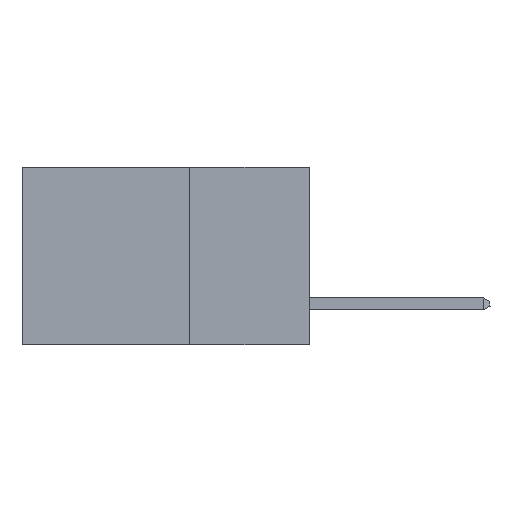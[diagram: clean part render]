
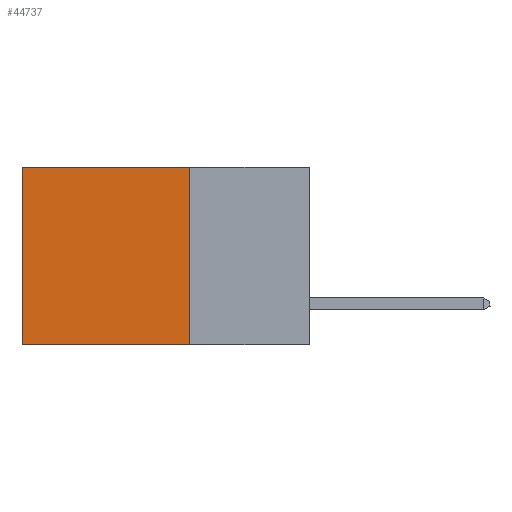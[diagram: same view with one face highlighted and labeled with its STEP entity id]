
A CAD part, left-side view. The second image highlights one B-rep face of the part: STEP entity #44737.
In plain terms, the highlighted planar face has unit normal (-1, 0, 0).
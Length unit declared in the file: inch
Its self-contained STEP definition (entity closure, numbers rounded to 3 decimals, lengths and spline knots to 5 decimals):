
#34 = VERTEX_POINT ( 'NONE', #30657 ) ;
#1559 = CARTESIAN_POINT ( 'NONE',  ( 0.2875, 0.25, 0. ) ) ;
#3124 = CARTESIAN_POINT ( 'NONE',  ( 0.2875, 0.6, -0.37 ) ) ;
#3145 = CARTESIAN_POINT ( 'NONE',  ( 0.2875, 0.6, 0. ) ) ;
#5218 = LINE ( 'NONE', #1559, #32919 ) ;
#6245 = VERTEX_POINT ( 'NONE', #25304 ) ;
#6445 = DIRECTION ( 'NONE',  ( 0., 0., -1. ) ) ;
#10493 = PLANE ( 'NONE',  #23070 ) ;
#14621 = DIRECTION ( 'NONE',  ( 1., 0., 0. ) ) ;
#14644 = DIRECTION ( 'NONE',  ( 0., 1., 0. ) ) ;
#15422 = VECTOR ( 'NONE', #6445, 39.37008 ) ;
#15622 = VECTOR ( 'NONE', #14644, 39.37008 ) ;
#15730 = ORIENTED_EDGE ( 'NONE', *, *, #23842, .F. ) ;
#17324 = CARTESIAN_POINT ( 'NONE',  ( 0.2875, 0.25, 0. ) ) ;
#18258 = CARTESIAN_POINT ( 'NONE',  ( 0.2875, 0.25, -0.37 ) ) ;
#18397 = DIRECTION ( 'NONE',  ( 0., 0., -1. ) ) ;
#21689 = ORIENTED_EDGE ( 'NONE', *, *, #38879, .F. ) ;
#21872 = LINE ( 'NONE', #29032, #15422 ) ;
#23070 = AXIS2_PLACEMENT_3D ( 'NONE', #37165, #14621, #18397 ) ;
#23842 = EDGE_CURVE ( 'NONE', #6245, #43455, #36805, .T. ) ;
#23954 = FACE_OUTER_BOUND ( 'NONE', #36875, .T. ) ;
#25304 = CARTESIAN_POINT ( 'NONE',  ( 0.2875, 0.25, -0.37 ) ) ;
#26646 = EDGE_CURVE ( 'NONE', #45426, #43455, #21872, .T. ) ;
#27005 = ORIENTED_EDGE ( 'NONE', *, *, #32850, .T. ) ;
#28950 = VECTOR ( 'NONE', #43688, 39.37008 ) ;
#29032 = CARTESIAN_POINT ( 'NONE',  ( 0.2875, 0.6, 0. ) ) ;
#30657 = CARTESIAN_POINT ( 'NONE',  ( 0.2875, 0.25, 0. ) ) ;
#32850 = EDGE_CURVE ( 'NONE', #34, #45426, #5218, .T. ) ;
#32919 = VECTOR ( 'NONE', #38872, 39.37008 ) ;
#36805 = LINE ( 'NONE', #18258, #15622 ) ;
#36875 = EDGE_LOOP ( 'NONE', ( #48639, #15730, #21689, #27005 ) ) ;
#37165 = CARTESIAN_POINT ( 'NONE',  ( 0.2875, 0.25, 0. ) ) ;
#38872 = DIRECTION ( 'NONE',  ( 0., 1., 0. ) ) ;
#38879 = EDGE_CURVE ( 'NONE', #34, #6245, #41923, .T. ) ;
#41923 = LINE ( 'NONE', #17324, #28950 ) ;
#43455 = VERTEX_POINT ( 'NONE', #3124 ) ;
#43688 = DIRECTION ( 'NONE',  ( 0., 0., -1. ) ) ;
#44737 = ADVANCED_FACE ( 'NONE', ( #23954 ), #10493, .F. ) ;
#45426 = VERTEX_POINT ( 'NONE', #3145 ) ;
#48639 = ORIENTED_EDGE ( 'NONE', *, *, #26646, .T. ) ;
